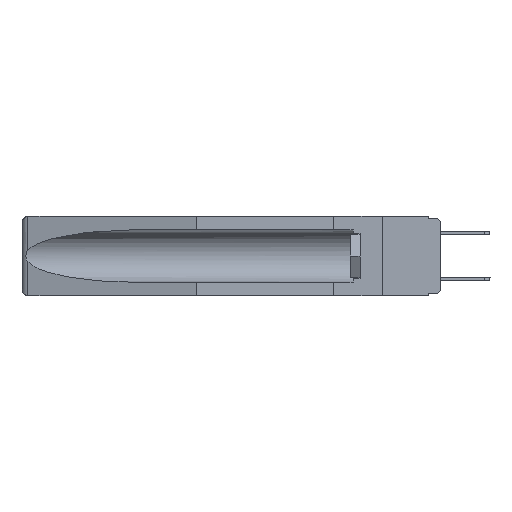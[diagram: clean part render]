
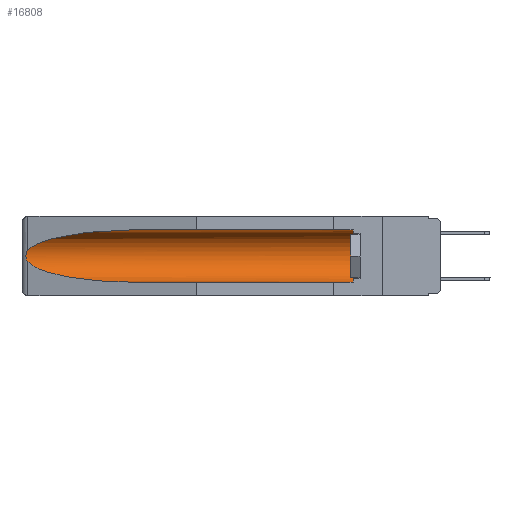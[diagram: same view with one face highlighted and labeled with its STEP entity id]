
A CAD part, left-side view. The second image highlights one B-rep face of the part: STEP entity #16808.
In plain terms, the highlighted cylindrical face has radius 2.857 mm (diameter 5.715 mm), a partial arc.
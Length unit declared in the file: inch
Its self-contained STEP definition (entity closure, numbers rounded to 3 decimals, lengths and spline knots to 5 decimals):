
#266 = EDGE_CURVE ( 'NONE', #957, #9468, #16066, .T. ) ;
#612 = VERTEX_POINT ( 'NONE', #2787 ) ;
#742 = CARTESIAN_POINT ( 'NONE',  ( 0.26597, 1.5296, -0.19026 ) ) ;
#957 = VERTEX_POINT ( 'NONE', #14656 ) ;
#1128 = CARTESIAN_POINT ( 'NONE',  ( 0.155, -0.30754, -0.059 ) ) ;
#1348 = CARTESIAN_POINT ( 'NONE',  ( 0.21114, 1.30732, -0.059 ) ) ;
#1673 = CIRCLE ( 'NONE', #2241, 0.1125 ) ;
#1684 = DIRECTION ( 'NONE',  ( 0., 1., 0. ) ) ;
#2241 = AXIS2_PLACEMENT_3D ( 'NONE', #7605, #3797, #7774 ) ;
#2583 = CARTESIAN_POINT ( 'NONE',  ( 0.26537, 1.52718, -0.19328 ) ) ;
#2787 = CARTESIAN_POINT ( 'NONE',  ( 0.155, 1.07973, -0.284 ) ) ;
#2874 = CARTESIAN_POINT ( 'NONE',  ( 0.26537, 1.52718, -0.14972 ) ) ;
#2983 = CARTESIAN_POINT ( 'NONE',  ( 0.155, 0.126, -0.284 ) ) ;
#3082 = EDGE_CURVE ( 'NONE', #13016, #957, #1673, .T. ) ;
#3502 = CARTESIAN_POINT ( 'NONE',  ( 0.26655, 1.53094, -0.18657 ) ) ;
#3797 = DIRECTION ( 'NONE',  ( 0., -1., 0. ) ) ;
#4087 = ORIENTED_EDGE ( 'NONE', *, *, #266, .T. ) ;
#4470 = CARTESIAN_POINT ( 'NONE',  ( 0.2673, 1.53269, -0.17917 ) ) ;
#4611 = CARTESIAN_POINT ( 'NONE',  ( 0.155, 1.07973, -0.059 ) ) ;
#4877 = DIRECTION ( 'NONE',  ( 0., 1., 0. ) ) ;
#5099 = B_SPLINE_CURVE_WITH_KNOTS ( 'NONE', 3,
 ( #9875, #16925, #15652, #14231, #7315, #8643, #4470, #3502, #742, #12640 ),
 .UNSPECIFIED., .F., .F.,
 ( 4, 2, 2, 2, 4 ),
 ( 0., 0.00029, 0.00058, 0.00087, 0.00117 ),
 .UNSPECIFIED. ) ;
#5223 = VERTEX_POINT ( 'NONE', #2583 ) ;
#5874 = DIRECTION ( 'NONE',  ( 0., 0., 1. ) ) ;
#5900 = VECTOR ( 'NONE', #6556, 39.37008 ) ;
#6204 = FACE_OUTER_BOUND ( 'NONE', #8749, .T. ) ;
#6448 = ORIENTED_EDGE ( 'NONE', *, *, #14059, .F. ) ;
#6556 = DIRECTION ( 'NONE',  ( 0., 1., 0. ) ) ;
#6789 =( BOUNDED_CURVE ( )  B_SPLINE_CURVE ( 3, ( #12923, #10409, #7591, #7676 ),
 .UNSPECIFIED., .F., .F. ) 
 B_SPLINE_CURVE_WITH_KNOTS ( ( 4, 4 ),
 ( 0.1948, 1.5708 ),
 .UNSPECIFIED. ) 
 CURVE ( )  GEOMETRIC_REPRESENTATION_ITEM ( )  RATIONAL_B_SPLINE_CURVE ( ( 1., 0.848, 0.848, 1. ) ) 
 REPRESENTATION_ITEM ( '' )  );
#7315 = CARTESIAN_POINT ( 'NONE',  ( 0.2675, 1.53308, -0.16763 ) ) ;
#7591 = CARTESIAN_POINT ( 'NONE',  ( 0.21114, 1.30732, -0.284 ) ) ;
#7605 = CARTESIAN_POINT ( 'NONE',  ( 0.155, 0.126, -0.1715 ) ) ;
#7676 = CARTESIAN_POINT ( 'NONE',  ( 0.155, 1.07973, -0.284 ) ) ;
#7746 = AXIS2_PLACEMENT_3D ( 'NONE', #8788, #4877, #5874 ) ;
#7774 = DIRECTION ( 'NONE',  ( 0., 0., 1. ) ) ;
#8612 =( BOUNDED_CURVE ( )  B_SPLINE_CURVE ( 3, ( #14947, #1348, #12363, #2874 ),
 .UNSPECIFIED., .F., .F. ) 
 B_SPLINE_CURVE_WITH_KNOTS ( ( 4, 4 ),
 ( 4.71239, 6.08839 ),
 .UNSPECIFIED. ) 
 CURVE ( )  GEOMETRIC_REPRESENTATION_ITEM ( )  RATIONAL_B_SPLINE_CURVE ( ( 1., 0.848, 0.848, 1. ) ) 
 REPRESENTATION_ITEM ( '' )  );
#8643 = CARTESIAN_POINT ( 'NONE',  ( 0.2675, 1.53308, -0.17534 ) ) ;
#8654 = EDGE_CURVE ( 'NONE', #14971, #5223, #5099, .T. ) ;
#8686 = ORIENTED_EDGE ( 'NONE', *, *, #11412, .T. ) ;
#8749 = EDGE_LOOP ( 'NONE', ( #15723, #11174, #8686, #6448, #15397, #4087 ) ) ;
#8788 = CARTESIAN_POINT ( 'NONE',  ( 0.155, -0.30754, -0.1715 ) ) ;
#9468 = VERTEX_POINT ( 'NONE', #4611 ) ;
#9875 = CARTESIAN_POINT ( 'NONE',  ( 0.26537, 1.52718, -0.14972 ) ) ;
#10409 = CARTESIAN_POINT ( 'NONE',  ( 0.25451, 1.48313, -0.24835 ) ) ;
#11174 = ORIENTED_EDGE ( 'NONE', *, *, #8654, .T. ) ;
#11268 = CARTESIAN_POINT ( 'NONE',  ( 0.155, -0.30754, -0.284 ) ) ;
#11412 = EDGE_CURVE ( 'NONE', #5223, #612, #6789, .T. ) ;
#11893 = CARTESIAN_POINT ( 'NONE',  ( 0.26537, 1.52718, -0.14972 ) ) ;
#12363 = CARTESIAN_POINT ( 'NONE',  ( 0.25451, 1.48313, -0.09465 ) ) ;
#12640 = CARTESIAN_POINT ( 'NONE',  ( 0.26537, 1.52718, -0.19328 ) ) ;
#12777 = VECTOR ( 'NONE', #1684, 39.37008 ) ;
#12923 = CARTESIAN_POINT ( 'NONE',  ( 0.26537, 1.52718, -0.19328 ) ) ;
#13016 = VERTEX_POINT ( 'NONE', #2983 ) ;
#13390 = EDGE_CURVE ( 'NONE', #9468, #14971, #8612, .T. ) ;
#13851 = LINE ( 'NONE', #11268, #12777 ) ;
#14059 = EDGE_CURVE ( 'NONE', #13016, #612, #13851, .T. ) ;
#14231 = CARTESIAN_POINT ( 'NONE',  ( 0.2673, 1.5327, -0.16383 ) ) ;
#14656 = CARTESIAN_POINT ( 'NONE',  ( 0.155, 0.126, -0.059 ) ) ;
#14947 = CARTESIAN_POINT ( 'NONE',  ( 0.155, 1.07973, -0.059 ) ) ;
#14971 = VERTEX_POINT ( 'NONE', #11893 ) ;
#15397 = ORIENTED_EDGE ( 'NONE', *, *, #3082, .T. ) ;
#15652 = CARTESIAN_POINT ( 'NONE',  ( 0.26654, 1.53092, -0.15636 ) ) ;
#15723 = ORIENTED_EDGE ( 'NONE', *, *, #13390, .T. ) ;
#16066 = LINE ( 'NONE', #1128, #5900 ) ;
#16808 = ADVANCED_FACE ( 'NONE', ( #6204 ), #16892, .F. ) ;
#16892 = CYLINDRICAL_SURFACE ( 'NONE', #7746, 0.1125 ) ;
#16925 = CARTESIAN_POINT ( 'NONE',  ( 0.26597, 1.52961, -0.15275 ) ) ;
